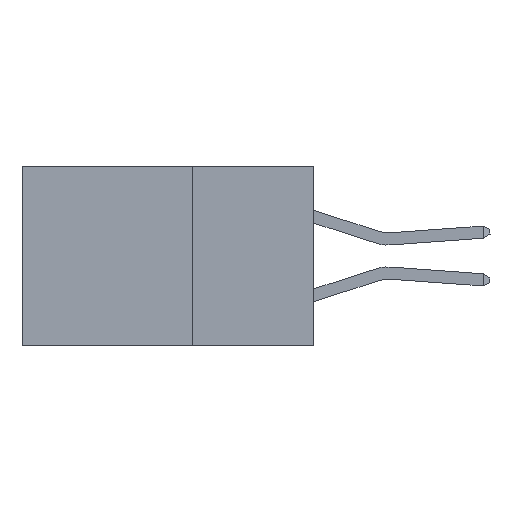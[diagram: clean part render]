
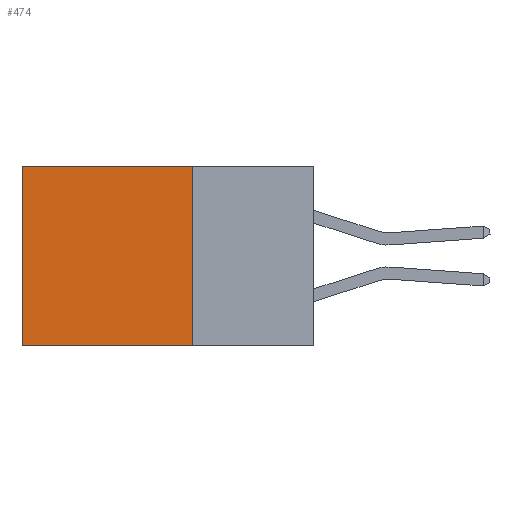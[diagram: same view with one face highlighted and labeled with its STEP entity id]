
A CAD part, left-side view. The second image highlights one B-rep face of the part: STEP entity #474.
In plain terms, the highlighted planar face has unit normal (-1, 0, 0).
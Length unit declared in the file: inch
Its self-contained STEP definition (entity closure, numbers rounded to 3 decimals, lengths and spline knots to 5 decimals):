
#67 = VECTOR ( 'NONE', #9102, 39.37008 ) ;
#180 = DIRECTION ( 'NONE',  ( 1., 0., 0. ) ) ;
#292 = LINE ( 'NONE', #11870, #11886 ) ;
#474 = ADVANCED_FACE ( 'NONE', ( #10618 ), #11418, .F. ) ;
#1470 = ORIENTED_EDGE ( 'NONE', *, *, #2823, .T. ) ;
#1730 = CARTESIAN_POINT ( 'NONE',  ( 0.2875, 0.25, 0. ) ) ;
#2526 = VERTEX_POINT ( 'NONE', #9465 ) ;
#2587 = CARTESIAN_POINT ( 'NONE',  ( 0.2875, 0.25, -0.37 ) ) ;
#2803 = AXIS2_PLACEMENT_3D ( 'NONE', #11460, #180, #3979 ) ;
#2823 = EDGE_CURVE ( 'NONE', #8628, #2526, #11606, .T. ) ;
#3142 = EDGE_LOOP ( 'NONE', ( #1470, #5054, #5237, #6089 ) ) ;
#3979 = DIRECTION ( 'NONE',  ( 0., 0., -1. ) ) ;
#4051 = DIRECTION ( 'NONE',  ( 0., 1., 0. ) ) ;
#4067 = VERTEX_POINT ( 'NONE', #1730 ) ;
#4110 = VECTOR ( 'NONE', #4051, 39.37008 ) ;
#4375 = DIRECTION ( 'NONE',  ( 0., 0., -1. ) ) ;
#4974 = VERTEX_POINT ( 'NONE', #9744 ) ;
#5054 = ORIENTED_EDGE ( 'NONE', *, *, #5075, .F. ) ;
#5075 = EDGE_CURVE ( 'NONE', #4974, #2526, #7858, .T. ) ;
#5225 = CARTESIAN_POINT ( 'NONE',  ( 0.2875, 0.6, 0. ) ) ;
#5237 = ORIENTED_EDGE ( 'NONE', *, *, #10726, .F. ) ;
#5732 = CARTESIAN_POINT ( 'NONE',  ( 0.2875, 0.6, 0. ) ) ;
#6089 = ORIENTED_EDGE ( 'NONE', *, *, #8698, .T. ) ;
#6746 = CARTESIAN_POINT ( 'NONE',  ( 0.2875, 0.25, 0. ) ) ;
#7858 = LINE ( 'NONE', #2587, #67 ) ;
#8628 = VERTEX_POINT ( 'NONE', #5732 ) ;
#8698 = EDGE_CURVE ( 'NONE', #4067, #8628, #8791, .T. ) ;
#8791 = LINE ( 'NONE', #6746, #4110 ) ;
#9102 = DIRECTION ( 'NONE',  ( 0., 1., 0. ) ) ;
#9132 = VECTOR ( 'NONE', #11778, 39.37008 ) ;
#9465 = CARTESIAN_POINT ( 'NONE',  ( 0.2875, 0.6, -0.37 ) ) ;
#9744 = CARTESIAN_POINT ( 'NONE',  ( 0.2875, 0.25, -0.37 ) ) ;
#10618 = FACE_OUTER_BOUND ( 'NONE', #3142, .T. ) ;
#10726 = EDGE_CURVE ( 'NONE', #4067, #4974, #292, .T. ) ;
#11418 = PLANE ( 'NONE',  #2803 ) ;
#11460 = CARTESIAN_POINT ( 'NONE',  ( 0.2875, 0.25, 0. ) ) ;
#11606 = LINE ( 'NONE', #5225, #9132 ) ;
#11778 = DIRECTION ( 'NONE',  ( 0., 0., -1. ) ) ;
#11870 = CARTESIAN_POINT ( 'NONE',  ( 0.2875, 0.25, 0. ) ) ;
#11886 = VECTOR ( 'NONE', #4375, 39.37008 ) ;
